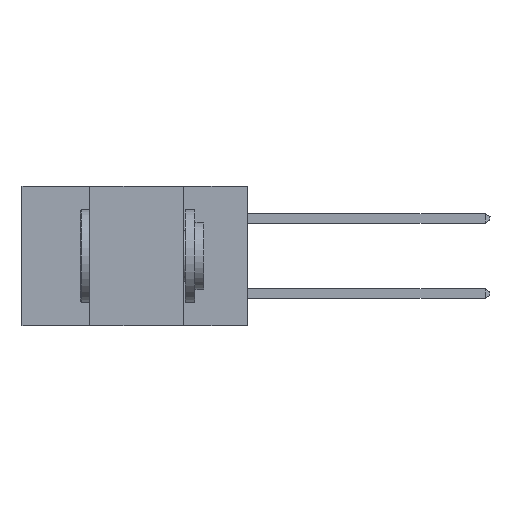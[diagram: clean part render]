
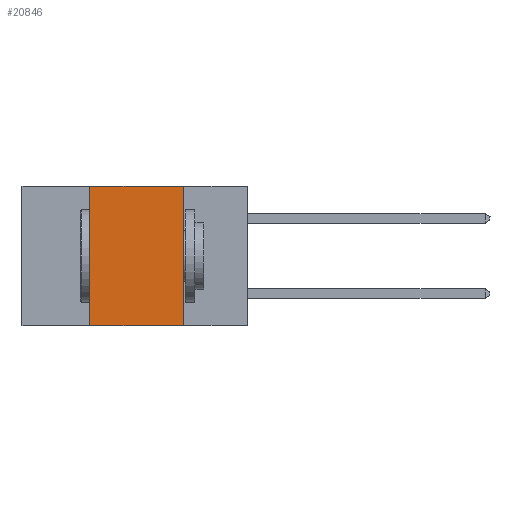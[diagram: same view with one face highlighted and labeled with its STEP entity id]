
A CAD part, left-side view. The second image highlights one B-rep face of the part: STEP entity #20846.
In plain terms, the highlighted planar face has unit normal (-1, 0, 0).
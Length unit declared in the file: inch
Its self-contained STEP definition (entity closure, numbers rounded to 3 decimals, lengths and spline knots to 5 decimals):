
#10 = ORIENTED_EDGE ( 'NONE', *, *, #18110, .T. ) ;
#643 = CARTESIAN_POINT ( 'NONE',  ( 0., 0.17, -0.37 ) ) ;
#2579 = PLANE ( 'NONE',  #9723 ) ;
#2848 = CARTESIAN_POINT ( 'NONE',  ( 0., 0.6, 0. ) ) ;
#6013 = LINE ( 'NONE', #16082, #13341 ) ;
#6972 = CARTESIAN_POINT ( 'NONE',  ( 0., 0.17, -0.37 ) ) ;
#7330 = LINE ( 'NONE', #13069, #19068 ) ;
#7365 = EDGE_CURVE ( 'NONE', #17069, #24084, #18145, .T. ) ;
#7704 = ORIENTED_EDGE ( 'NONE', *, *, #7365, .F. ) ;
#8174 = DIRECTION ( 'NONE',  ( 0., 0., 1. ) ) ;
#8431 = DIRECTION ( 'NONE',  ( 0., 0., -1. ) ) ;
#9723 = AXIS2_PLACEMENT_3D ( 'NONE', #2848, #18435, #10373 ) ;
#10373 = DIRECTION ( 'NONE',  ( 0., 0., -1. ) ) ;
#11606 = CARTESIAN_POINT ( 'NONE',  ( 0., 0.42, -0.37 ) ) ;
#12891 = VERTEX_POINT ( 'NONE', #11606 ) ;
#13069 = CARTESIAN_POINT ( 'NONE',  ( 0., 0.6, 0. ) ) ;
#13334 = VECTOR ( 'NONE', #8431, 39.37008 ) ;
#13341 = VECTOR ( 'NONE', #8174, 39.37008 ) ;
#14457 = FACE_OUTER_BOUND ( 'NONE', #18832, .T. ) ;
#16029 = ORIENTED_EDGE ( 'NONE', *, *, #19163, .F. ) ;
#16082 = CARTESIAN_POINT ( 'NONE',  ( 0., 0.42, -0.37 ) ) ;
#17069 = VERTEX_POINT ( 'NONE', #22822 ) ;
#17147 = EDGE_CURVE ( 'NONE', #23454, #17069, #7330, .T. ) ;
#17223 = DIRECTION ( 'NONE',  ( 0., -1., 0. ) ) ;
#17286 = DIRECTION ( 'NONE',  ( 0., -1., 0. ) ) ;
#18110 = EDGE_CURVE ( 'NONE', #12891, #24084, #19273, .T. ) ;
#18145 = LINE ( 'NONE', #643, #13334 ) ;
#18435 = DIRECTION ( 'NONE',  ( 1., 0., 0. ) ) ;
#18832 = EDGE_LOOP ( 'NONE', ( #7704, #24870, #16029, #10 ) ) ;
#19068 = VECTOR ( 'NONE', #17286, 39.37008 ) ;
#19148 = CARTESIAN_POINT ( 'NONE',  ( 0., 0.6, -0.37 ) ) ;
#19163 = EDGE_CURVE ( 'NONE', #12891, #23454, #6013, .T. ) ;
#19273 = LINE ( 'NONE', #19148, #21952 ) ;
#20846 = ADVANCED_FACE ( 'NONE', ( #14457 ), #2579, .F. ) ;
#21952 = VECTOR ( 'NONE', #17223, 39.37008 ) ;
#22228 = CARTESIAN_POINT ( 'NONE',  ( 0., 0.42, 0. ) ) ;
#22822 = CARTESIAN_POINT ( 'NONE',  ( 0., 0.17, 0. ) ) ;
#23454 = VERTEX_POINT ( 'NONE', #22228 ) ;
#24084 = VERTEX_POINT ( 'NONE', #6972 ) ;
#24870 = ORIENTED_EDGE ( 'NONE', *, *, #17147, .F. ) ;
